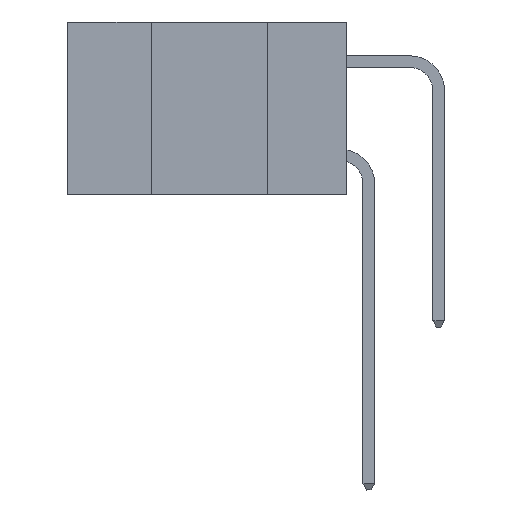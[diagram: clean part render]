
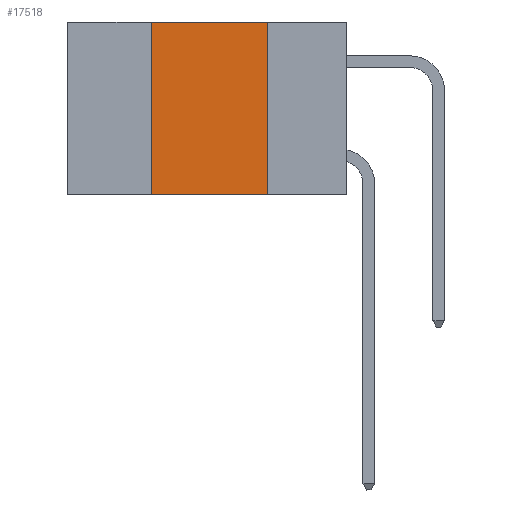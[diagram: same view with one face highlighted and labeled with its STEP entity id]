
A CAD part, left-side view. The second image highlights one B-rep face of the part: STEP entity #17518.
In plain terms, the highlighted planar face has unit normal (-1, 0, 0).
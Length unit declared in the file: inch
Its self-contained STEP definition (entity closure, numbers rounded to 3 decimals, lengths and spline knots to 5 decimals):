
#1299 = LINE ( 'NONE', #18124, #1843 ) ;
#1346 = LINE ( 'NONE', #13755, #19624 ) ;
#1843 = VECTOR ( 'NONE', #19924, 39.37008 ) ;
#1902 = EDGE_CURVE ( 'NONE', #12215, #11882, #21671, .T. ) ;
#2381 = CARTESIAN_POINT ( 'NONE',  ( 0., 0.42, 0. ) ) ;
#2486 = DIRECTION ( 'NONE',  ( 1., 0., 0. ) ) ;
#2648 = CARTESIAN_POINT ( 'NONE',  ( 0., 0.6, 0. ) ) ;
#3162 = VECTOR ( 'NONE', #15506, 39.37008 ) ;
#5508 = EDGE_CURVE ( 'NONE', #11882, #19567, #12527, .T. ) ;
#6749 = FACE_OUTER_BOUND ( 'NONE', #16347, .T. ) ;
#7259 = CARTESIAN_POINT ( 'NONE',  ( 0., 0.42, -0.37 ) ) ;
#7952 = DIRECTION ( 'NONE',  ( 0., 0., -1. ) ) ;
#8349 = CARTESIAN_POINT ( 'NONE',  ( 0., 0.17, 0. ) ) ;
#8418 = DIRECTION ( 'NONE',  ( 0., -1., 0. ) ) ;
#8864 = ORIENTED_EDGE ( 'NONE', *, *, #19308, .F. ) ;
#10776 = ORIENTED_EDGE ( 'NONE', *, *, #16192, .T. ) ;
#11311 = PLANE ( 'NONE',  #13417 ) ;
#11882 = VERTEX_POINT ( 'NONE', #21379 ) ;
#12215 = VERTEX_POINT ( 'NONE', #2381 ) ;
#12527 = LINE ( 'NONE', #8349, #3162 ) ;
#13417 = AXIS2_PLACEMENT_3D ( 'NONE', #2648, #2486, #7952 ) ;
#13755 = CARTESIAN_POINT ( 'NONE',  ( 0., 0.42, 0. ) ) ;
#13783 = ORIENTED_EDGE ( 'NONE', *, *, #1902, .F. ) ;
#14733 = CARTESIAN_POINT ( 'NONE',  ( 0., 0.17, -0.37 ) ) ;
#15506 = DIRECTION ( 'NONE',  ( 0., 0., -1. ) ) ;
#16192 = EDGE_CURVE ( 'NONE', #20653, #19567, #1299, .T. ) ;
#16347 = EDGE_LOOP ( 'NONE', ( #19792, #13783, #8864, #10776 ) ) ;
#16933 = VECTOR ( 'NONE', #8418, 39.37008 ) ;
#17518 = ADVANCED_FACE ( 'NONE', ( #6749 ), #11311, .F. ) ;
#18124 = CARTESIAN_POINT ( 'NONE',  ( 0., 0.6, -0.37 ) ) ;
#19122 = CARTESIAN_POINT ( 'NONE',  ( 0., 0.6, 0. ) ) ;
#19308 = EDGE_CURVE ( 'NONE', #20653, #12215, #1346, .T. ) ;
#19567 = VERTEX_POINT ( 'NONE', #14733 ) ;
#19624 = VECTOR ( 'NONE', #20896, 39.37008 ) ;
#19792 = ORIENTED_EDGE ( 'NONE', *, *, #5508, .F. ) ;
#19924 = DIRECTION ( 'NONE',  ( 0., -1., 0. ) ) ;
#20653 = VERTEX_POINT ( 'NONE', #7259 ) ;
#20896 = DIRECTION ( 'NONE',  ( 0., 0., 1. ) ) ;
#21379 = CARTESIAN_POINT ( 'NONE',  ( 0., 0.17, 0. ) ) ;
#21671 = LINE ( 'NONE', #19122, #16933 ) ;
